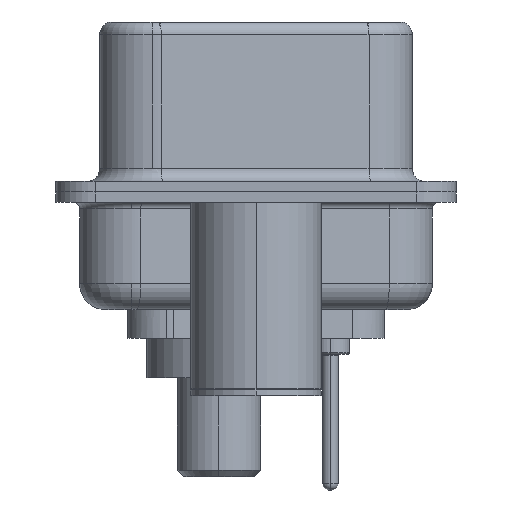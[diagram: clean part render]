
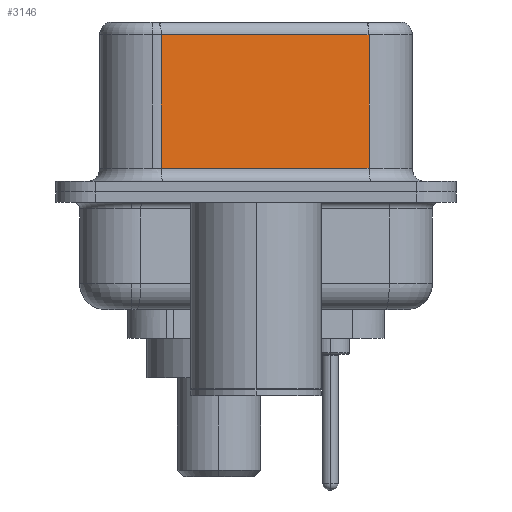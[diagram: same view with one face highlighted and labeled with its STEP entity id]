
A CAD part, left-side view. The second image highlights one B-rep face of the part: STEP entity #3146.
In plain terms, the highlighted planar face has unit normal (-0.985, -0.174, 0).
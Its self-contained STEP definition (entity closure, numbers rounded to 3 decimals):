
#178 = AXIS2_PLACEMENT_3D ( 'NONE', #23464, #16793, #19605 ) ;
#689 = PLANE ( 'NONE',  #178 ) ;
#720 = VECTOR ( 'NONE', #18602, 1000. ) ;
#760 = LINE ( 'NONE', #19586, #15883 ) ;
#3146 = ADVANCED_FACE ( 'NONE', ( #11124 ), #689, .F. ) ;
#4076 = VECTOR ( 'NONE', #23811, 1000. ) ;
#4651 = EDGE_CURVE ( 'NONE', #4782, #4828, #20589, .T. ) ;
#4782 = VERTEX_POINT ( 'NONE', #22859 ) ;
#4828 = VERTEX_POINT ( 'NONE', #14178 ) ;
#5749 = VERTEX_POINT ( 'NONE', #9767 ) ;
#6016 = ORIENTED_EDGE ( 'NONE', *, *, #24627, .F. ) ;
#8308 = VERTEX_POINT ( 'NONE', #24818 ) ;
#8822 = ORIENTED_EDGE ( 'NONE', *, *, #4651, .T. ) ;
#9296 = LINE ( 'NONE', #21839, #4076 ) ;
#9767 = CARTESIAN_POINT ( 'NONE',  ( 3.73, 3.628, 0.9 ) ) ;
#11124 = FACE_OUTER_BOUND ( 'NONE', #14261, .T. ) ;
#11648 = DIRECTION ( 'NONE',  ( -0.174, 0.985, 0. ) ) ;
#11869 = EDGE_CURVE ( 'NONE', #5749, #8308, #9296, .T. ) ;
#12424 = ORIENTED_EDGE ( 'NONE', *, *, #18137, .T. ) ;
#14178 = CARTESIAN_POINT ( 'NONE',  ( 3.73, 3.628, 6.02 ) ) ;
#14261 = EDGE_LOOP ( 'NONE', ( #6016, #8822, #12424, #15776 ) ) ;
#15402 = VECTOR ( 'NONE', #11648, 1000. ) ;
#15776 = ORIENTED_EDGE ( 'NONE', *, *, #11869, .T. ) ;
#15883 = VECTOR ( 'NONE', #21465, 1000. ) ;
#16625 = CARTESIAN_POINT ( 'NONE',  ( 3.73, 3.628, 6.52 ) ) ;
#16793 = DIRECTION ( 'NONE',  ( 0.985, 0.174, 0. ) ) ;
#18137 = EDGE_CURVE ( 'NONE', #4828, #5749, #21645, .T. ) ;
#18602 = DIRECTION ( 'NONE',  ( 0., 0., -1. ) ) ;
#19431 = CARTESIAN_POINT ( 'NONE',  ( 5.132, -4.322, 6.02 ) ) ;
#19586 = CARTESIAN_POINT ( 'NONE',  ( 5.132, -4.322, 6.52 ) ) ;
#19605 = DIRECTION ( 'NONE',  ( -0.174, 0.985, 0. ) ) ;
#20589 = LINE ( 'NONE', #19431, #15402 ) ;
#21465 = DIRECTION ( 'NONE',  ( 0., 0., -1. ) ) ;
#21645 = LINE ( 'NONE', #16625, #720 ) ;
#21839 = CARTESIAN_POINT ( 'NONE',  ( 5.132, -4.322, 0.9 ) ) ;
#22859 = CARTESIAN_POINT ( 'NONE',  ( 5.132, -4.322, 6.02 ) ) ;
#23464 = CARTESIAN_POINT ( 'NONE',  ( 5.132, -4.322, 6.52 ) ) ;
#23811 = DIRECTION ( 'NONE',  ( 0.174, -0.985, 0. ) ) ;
#24627 = EDGE_CURVE ( 'NONE', #4782, #8308, #760, .T. ) ;
#24818 = CARTESIAN_POINT ( 'NONE',  ( 5.132, -4.322, 0.9 ) ) ;
